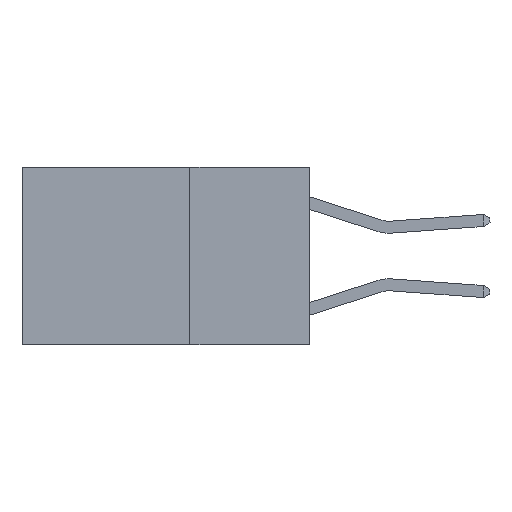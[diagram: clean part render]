
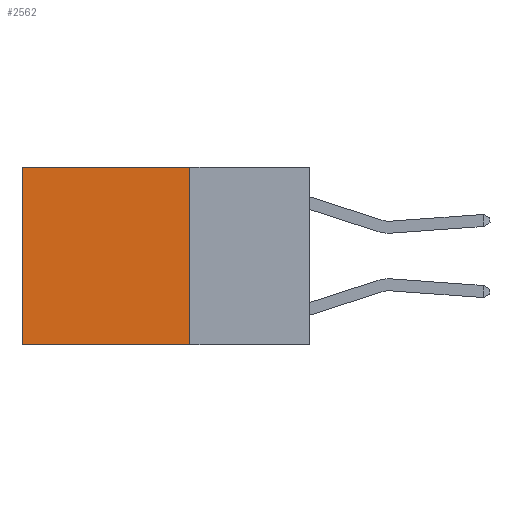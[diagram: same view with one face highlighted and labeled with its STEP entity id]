
A CAD part, left-side view. The second image highlights one B-rep face of the part: STEP entity #2562.
In plain terms, the highlighted planar face has unit normal (-1, 0, 0).
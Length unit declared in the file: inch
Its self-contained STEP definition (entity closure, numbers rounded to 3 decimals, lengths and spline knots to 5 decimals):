
#312 = CARTESIAN_POINT ( 'NONE',  ( 0.2625, 0.25, 0. ) ) ;
#536 = LINE ( 'NONE', #3142, #4717 ) ;
#633 = DIRECTION ( 'NONE',  ( 0., 0., -1. ) ) ;
#1068 = VECTOR ( 'NONE', #2025, 39.37008 ) ;
#1298 = CARTESIAN_POINT ( 'NONE',  ( 0.2625, 0.6, 0. ) ) ;
#1442 = VERTEX_POINT ( 'NONE', #7704 ) ;
#1778 = DIRECTION ( 'NONE',  ( 0., 0., -1. ) ) ;
#1864 = EDGE_CURVE ( 'NONE', #5436, #5033, #3795, .T. ) ;
#1945 = CARTESIAN_POINT ( 'NONE',  ( 0.2625, 0.25, -0.37 ) ) ;
#2025 = DIRECTION ( 'NONE',  ( 0., 1., 0. ) ) ;
#2311 = LINE ( 'NONE', #10463, #6423 ) ;
#2562 = ADVANCED_FACE ( 'NONE', ( #9907 ), #7223, .F. ) ;
#2576 = CARTESIAN_POINT ( 'NONE',  ( 0.2625, 0.6, 0. ) ) ;
#3080 = EDGE_CURVE ( 'NONE', #1442, #4051, #2311, .T. ) ;
#3142 = CARTESIAN_POINT ( 'NONE',  ( 0.2625, 0.25, -0.37 ) ) ;
#3149 = DIRECTION ( 'NONE',  ( 1., 0., 0. ) ) ;
#3174 = AXIS2_PLACEMENT_3D ( 'NONE', #8028, #3149, #8853 ) ;
#3795 = LINE ( 'NONE', #2576, #10040 ) ;
#3996 = ORIENTED_EDGE ( 'NONE', *, *, #1864, .T. ) ;
#4051 = VERTEX_POINT ( 'NONE', #1945 ) ;
#4717 = VECTOR ( 'NONE', #10530, 39.37008 ) ;
#4762 = ORIENTED_EDGE ( 'NONE', *, *, #6712, .T. ) ;
#5033 = VERTEX_POINT ( 'NONE', #8083 ) ;
#5197 = LINE ( 'NONE', #312, #1068 ) ;
#5436 = VERTEX_POINT ( 'NONE', #1298 ) ;
#6165 = ORIENTED_EDGE ( 'NONE', *, *, #6292, .F. ) ;
#6292 = EDGE_CURVE ( 'NONE', #4051, #5033, #536, .T. ) ;
#6423 = VECTOR ( 'NONE', #633, 39.37008 ) ;
#6712 = EDGE_CURVE ( 'NONE', #1442, #5436, #5197, .T. ) ;
#7223 = PLANE ( 'NONE',  #3174 ) ;
#7704 = CARTESIAN_POINT ( 'NONE',  ( 0.2625, 0.25, 0. ) ) ;
#8028 = CARTESIAN_POINT ( 'NONE',  ( 0.2625, 0.25, 0. ) ) ;
#8083 = CARTESIAN_POINT ( 'NONE',  ( 0.2625, 0.6, -0.37 ) ) ;
#8591 = ORIENTED_EDGE ( 'NONE', *, *, #3080, .F. ) ;
#8853 = DIRECTION ( 'NONE',  ( 0., 0., -1. ) ) ;
#8953 = EDGE_LOOP ( 'NONE', ( #3996, #6165, #8591, #4762 ) ) ;
#9907 = FACE_OUTER_BOUND ( 'NONE', #8953, .T. ) ;
#10040 = VECTOR ( 'NONE', #1778, 39.37008 ) ;
#10463 = CARTESIAN_POINT ( 'NONE',  ( 0.2625, 0.25, 0. ) ) ;
#10530 = DIRECTION ( 'NONE',  ( 0., 1., 0. ) ) ;
